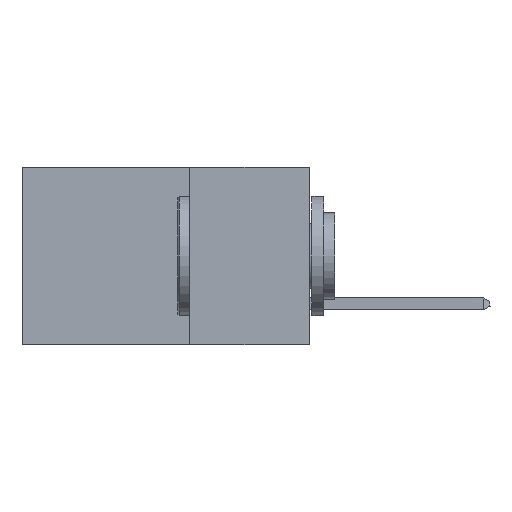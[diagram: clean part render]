
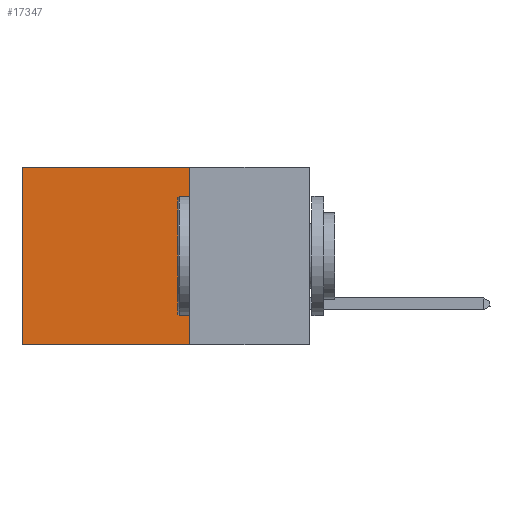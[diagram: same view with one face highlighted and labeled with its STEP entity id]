
A CAD part, left-side view. The second image highlights one B-rep face of the part: STEP entity #17347.
In plain terms, the highlighted planar face has unit normal (-1, 0, 0).
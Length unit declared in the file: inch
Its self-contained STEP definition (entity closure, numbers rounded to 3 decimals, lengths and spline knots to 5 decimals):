
#149 = VERTEX_POINT ( 'NONE', #6166 ) ;
#242 = CARTESIAN_POINT ( 'NONE',  ( 0.2875, 0.6, 0. ) ) ;
#328 = EDGE_CURVE ( 'NONE', #13449, #5590, #10627, .T. ) ;
#2316 = AXIS2_PLACEMENT_3D ( 'NONE', #18592, #21326, #7268 ) ;
#2946 = LINE ( 'NONE', #3075, #24647 ) ;
#3075 = CARTESIAN_POINT ( 'NONE',  ( 0.2875, 0.25, 0. ) ) ;
#3768 = LINE ( 'NONE', #27056, #25088 ) ;
#5590 = VERTEX_POINT ( 'NONE', #17030 ) ;
#5796 = CARTESIAN_POINT ( 'NONE',  ( 0.2875, 0.25, 0. ) ) ;
#6166 = CARTESIAN_POINT ( 'NONE',  ( 0.2875, 0.6, -0.37 ) ) ;
#7268 = DIRECTION ( 'NONE',  ( 0., 0., -1. ) ) ;
#7422 = ORIENTED_EDGE ( 'NONE', *, *, #22588, .T. ) ;
#7816 = DIRECTION ( 'NONE',  ( 0., 1., 0. ) ) ;
#8464 = DIRECTION ( 'NONE',  ( 0., 0., -1. ) ) ;
#9616 = LINE ( 'NONE', #28565, #14387 ) ;
#10627 = LINE ( 'NONE', #5796, #18390 ) ;
#11485 = CARTESIAN_POINT ( 'NONE',  ( 0.2875, 0.25, 0. ) ) ;
#13449 = VERTEX_POINT ( 'NONE', #11485 ) ;
#14387 = VECTOR ( 'NONE', #14509, 39.37008 ) ;
#14509 = DIRECTION ( 'NONE',  ( 0., 1., 0. ) ) ;
#16552 = ORIENTED_EDGE ( 'NONE', *, *, #26052, .T. ) ;
#16779 = ORIENTED_EDGE ( 'NONE', *, *, #25972, .F. ) ;
#17030 = CARTESIAN_POINT ( 'NONE',  ( 0.2875, 0.25, -0.37 ) ) ;
#17347 = ADVANCED_FACE ( 'NONE', ( #19008 ), #19198, .F. ) ;
#18390 = VECTOR ( 'NONE', #24891, 39.37008 ) ;
#18592 = CARTESIAN_POINT ( 'NONE',  ( 0.2875, 0.25, 0. ) ) ;
#19008 = FACE_OUTER_BOUND ( 'NONE', #22861, .T. ) ;
#19198 = PLANE ( 'NONE',  #2316 ) ;
#20981 = VERTEX_POINT ( 'NONE', #242 ) ;
#21326 = DIRECTION ( 'NONE',  ( 1., 0., 0. ) ) ;
#22588 = EDGE_CURVE ( 'NONE', #20981, #149, #3768, .T. ) ;
#22861 = EDGE_LOOP ( 'NONE', ( #7422, #16779, #26369, #16552 ) ) ;
#24647 = VECTOR ( 'NONE', #7816, 39.37008 ) ;
#24891 = DIRECTION ( 'NONE',  ( 0., 0., -1. ) ) ;
#25088 = VECTOR ( 'NONE', #8464, 39.37008 ) ;
#25972 = EDGE_CURVE ( 'NONE', #5590, #149, #9616, .T. ) ;
#26052 = EDGE_CURVE ( 'NONE', #13449, #20981, #2946, .T. ) ;
#26369 = ORIENTED_EDGE ( 'NONE', *, *, #328, .F. ) ;
#27056 = CARTESIAN_POINT ( 'NONE',  ( 0.2875, 0.6, 0. ) ) ;
#28565 = CARTESIAN_POINT ( 'NONE',  ( 0.2875, 0.25, -0.37 ) ) ;
